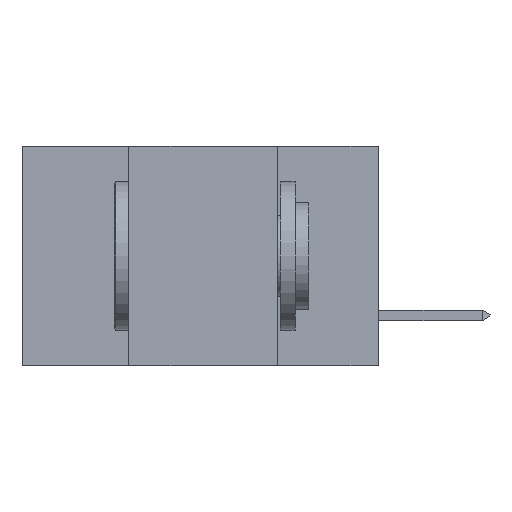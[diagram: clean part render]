
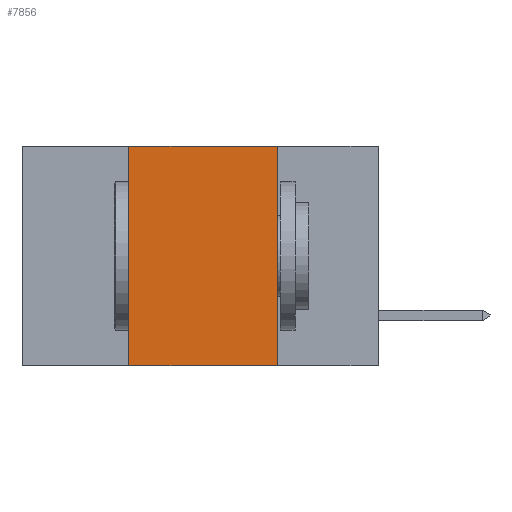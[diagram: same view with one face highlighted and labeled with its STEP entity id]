
A CAD part, left-side view. The second image highlights one B-rep face of the part: STEP entity #7856.
In plain terms, the highlighted planar face has unit normal (-1, 0, 0).
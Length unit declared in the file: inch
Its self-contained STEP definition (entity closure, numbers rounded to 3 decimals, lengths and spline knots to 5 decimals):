
#251 = CARTESIAN_POINT ( 'NONE',  ( 0., 0.6, -0.37 ) ) ;
#556 = LINE ( 'NONE', #16963, #6436 ) ;
#1312 = LINE ( 'NONE', #10305, #16765 ) ;
#1745 = EDGE_CURVE ( 'NONE', #12621, #21333, #1312, .T. ) ;
#1889 = EDGE_CURVE ( 'NONE', #9470, #20436, #556, .T. ) ;
#2301 = CARTESIAN_POINT ( 'NONE',  ( 0., 0.42, 0. ) ) ;
#2948 = AXIS2_PLACEMENT_3D ( 'NONE', #4038, #7505, #13135 ) ;
#4038 = CARTESIAN_POINT ( 'NONE',  ( 0., 0.6, 0. ) ) ;
#4302 = CARTESIAN_POINT ( 'NONE',  ( 0., 0.42, -0.37 ) ) ;
#6436 = VECTOR ( 'NONE', #18530, 39.37008 ) ;
#7505 = DIRECTION ( 'NONE',  ( 1., 0., 0. ) ) ;
#7675 = DIRECTION ( 'NONE',  ( 0., -1., 0. ) ) ;
#7856 = ADVANCED_FACE ( 'NONE', ( #16967 ), #11232, .F. ) ;
#7864 = LINE ( 'NONE', #13495, #13843 ) ;
#8300 = VECTOR ( 'NONE', #7675, 39.37008 ) ;
#9068 = EDGE_CURVE ( 'NONE', #9470, #21333, #13190, .T. ) ;
#9427 = DIRECTION ( 'NONE',  ( 0., -1., 0. ) ) ;
#9470 = VERTEX_POINT ( 'NONE', #4302 ) ;
#10305 = CARTESIAN_POINT ( 'NONE',  ( 0., 0.17, -0.37 ) ) ;
#11232 = PLANE ( 'NONE',  #2948 ) ;
#12621 = VERTEX_POINT ( 'NONE', #13271 ) ;
#13135 = DIRECTION ( 'NONE',  ( 0., 0., -1. ) ) ;
#13190 = LINE ( 'NONE', #251, #8300 ) ;
#13271 = CARTESIAN_POINT ( 'NONE',  ( 0., 0.17, 0. ) ) ;
#13495 = CARTESIAN_POINT ( 'NONE',  ( 0., 0.6, 0. ) ) ;
#13843 = VECTOR ( 'NONE', #9427, 39.37008 ) ;
#15394 = ORIENTED_EDGE ( 'NONE', *, *, #1745, .F. ) ;
#15564 = ORIENTED_EDGE ( 'NONE', *, *, #20829, .F. ) ;
#16765 = VECTOR ( 'NONE', #21586, 39.37008 ) ;
#16963 = CARTESIAN_POINT ( 'NONE',  ( 0., 0.42, -0.37 ) ) ;
#16967 = FACE_OUTER_BOUND ( 'NONE', #22530, .T. ) ;
#17573 = ORIENTED_EDGE ( 'NONE', *, *, #9068, .T. ) ;
#18530 = DIRECTION ( 'NONE',  ( 0., 0., 1. ) ) ;
#18628 = CARTESIAN_POINT ( 'NONE',  ( 0., 0.17, -0.37 ) ) ;
#20219 = ORIENTED_EDGE ( 'NONE', *, *, #1889, .F. ) ;
#20436 = VERTEX_POINT ( 'NONE', #2301 ) ;
#20829 = EDGE_CURVE ( 'NONE', #20436, #12621, #7864, .T. ) ;
#21333 = VERTEX_POINT ( 'NONE', #18628 ) ;
#21586 = DIRECTION ( 'NONE',  ( 0., 0., -1. ) ) ;
#22530 = EDGE_LOOP ( 'NONE', ( #15394, #15564, #20219, #17573 ) ) ;
